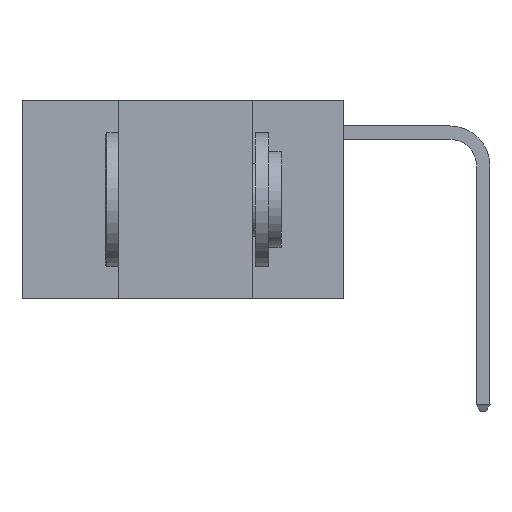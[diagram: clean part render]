
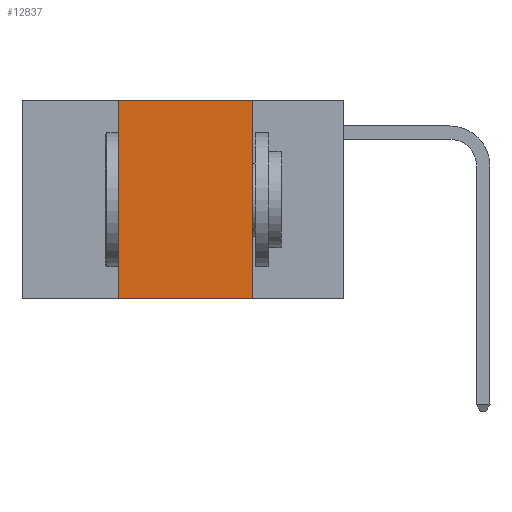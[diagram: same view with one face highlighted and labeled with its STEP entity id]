
A CAD part, left-side view. The second image highlights one B-rep face of the part: STEP entity #12837.
In plain terms, the highlighted planar face has unit normal (-1, 0, 0).
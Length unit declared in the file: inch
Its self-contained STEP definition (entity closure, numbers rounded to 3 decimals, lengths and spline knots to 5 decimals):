
#606 = DIRECTION ( 'NONE',  ( 0., -1., 0. ) ) ;
#1314 = LINE ( 'NONE', #20617, #13304 ) ;
#1435 = CARTESIAN_POINT ( 'NONE',  ( 0., 0.6, 0. ) ) ;
#2081 = CARTESIAN_POINT ( 'NONE',  ( 0., 0.6, -0.37 ) ) ;
#2850 = DIRECTION ( 'NONE',  ( 0., 0., -1. ) ) ;
#3095 = DIRECTION ( 'NONE',  ( 1., 0., 0. ) ) ;
#3187 = ORIENTED_EDGE ( 'NONE', *, *, #15007, .F. ) ;
#5600 = ORIENTED_EDGE ( 'NONE', *, *, #22353, .F. ) ;
#6921 = EDGE_CURVE ( 'NONE', #11232, #12398, #1314, .T. ) ;
#7494 = VERTEX_POINT ( 'NONE', #13661 ) ;
#8142 = VERTEX_POINT ( 'NONE', #13562 ) ;
#8302 = DIRECTION ( 'NONE',  ( 0., 0., 1. ) ) ;
#8481 = ORIENTED_EDGE ( 'NONE', *, *, #6921, .F. ) ;
#8822 = AXIS2_PLACEMENT_3D ( 'NONE', #12595, #3095, #2850 ) ;
#10739 = CARTESIAN_POINT ( 'NONE',  ( 0., 0.17, -0.37 ) ) ;
#11232 = VERTEX_POINT ( 'NONE', #23830 ) ;
#12066 = DIRECTION ( 'NONE',  ( 0., -1., 0. ) ) ;
#12398 = VERTEX_POINT ( 'NONE', #10739 ) ;
#12595 = CARTESIAN_POINT ( 'NONE',  ( 0., 0.6, 0. ) ) ;
#12837 = ADVANCED_FACE ( 'NONE', ( #18012 ), #17892, .F. ) ;
#13304 = VECTOR ( 'NONE', #16575, 39.37008 ) ;
#13562 = CARTESIAN_POINT ( 'NONE',  ( 0., 0.42, 0. ) ) ;
#13661 = CARTESIAN_POINT ( 'NONE',  ( 0., 0.42, -0.37 ) ) ;
#14172 = CARTESIAN_POINT ( 'NONE',  ( 0., 0.42, 0. ) ) ;
#15007 = EDGE_CURVE ( 'NONE', #7494, #8142, #17836, .T. ) ;
#16575 = DIRECTION ( 'NONE',  ( 0., 0., -1. ) ) ;
#16647 = EDGE_LOOP ( 'NONE', ( #8481, #5600, #3187, #19610 ) ) ;
#16777 = VECTOR ( 'NONE', #12066, 39.37008 ) ;
#17480 = LINE ( 'NONE', #2081, #16777 ) ;
#17836 = LINE ( 'NONE', #14172, #20997 ) ;
#17892 = PLANE ( 'NONE',  #8822 ) ;
#18012 = FACE_OUTER_BOUND ( 'NONE', #16647, .T. ) ;
#18719 = LINE ( 'NONE', #1435, #20422 ) ;
#19610 = ORIENTED_EDGE ( 'NONE', *, *, #24504, .T. ) ;
#20422 = VECTOR ( 'NONE', #606, 39.37008 ) ;
#20617 = CARTESIAN_POINT ( 'NONE',  ( 0., 0.17, 0. ) ) ;
#20997 = VECTOR ( 'NONE', #8302, 39.37008 ) ;
#22353 = EDGE_CURVE ( 'NONE', #8142, #11232, #18719, .T. ) ;
#23830 = CARTESIAN_POINT ( 'NONE',  ( 0., 0.17, 0. ) ) ;
#24504 = EDGE_CURVE ( 'NONE', #7494, #12398, #17480, .T. ) ;
